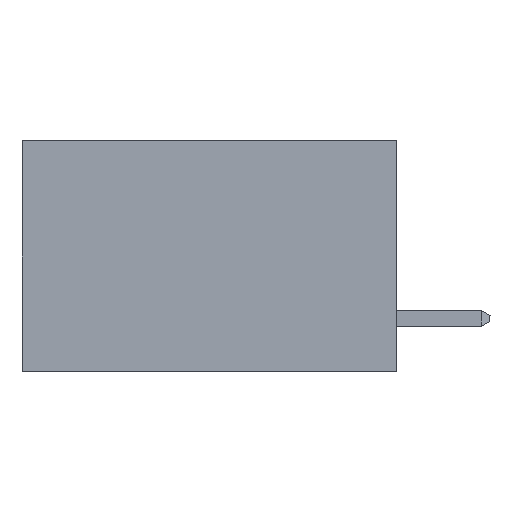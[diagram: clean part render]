
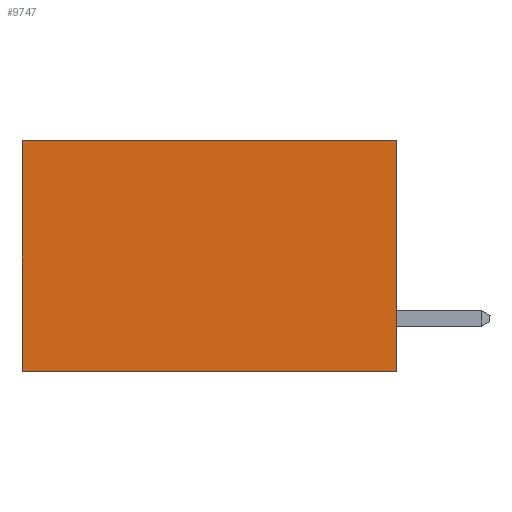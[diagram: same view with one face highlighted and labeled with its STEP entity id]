
A CAD part, left-side view. The second image highlights one B-rep face of the part: STEP entity #9747.
In plain terms, the highlighted planar face has unit normal (-1, 0, 0).
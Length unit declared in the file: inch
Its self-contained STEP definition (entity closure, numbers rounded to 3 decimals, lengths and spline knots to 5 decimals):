
#568 = PLANE ( 'NONE',  #11723 ) ;
#1338 = CARTESIAN_POINT ( 'NONE',  ( 0.2615, 0., -0.37 ) ) ;
#1835 = CARTESIAN_POINT ( 'NONE',  ( 0.2615, 0., -0.37 ) ) ;
#3425 = LINE ( 'NONE', #9785, #19022 ) ;
#3482 = EDGE_LOOP ( 'NONE', ( #17661, #17307, #8481, #19123 ) ) ;
#3510 = LINE ( 'NONE', #19877, #14342 ) ;
#6189 = LINE ( 'NONE', #20429, #20233 ) ;
#7108 = DIRECTION ( 'NONE',  ( 0., 0., -1. ) ) ;
#7297 = LINE ( 'NONE', #16811, #17138 ) ;
#7397 = DIRECTION ( 'NONE',  ( 0., 1., 0. ) ) ;
#8481 = ORIENTED_EDGE ( 'NONE', *, *, #20090, .F. ) ;
#8955 = CARTESIAN_POINT ( 'NONE',  ( 0.2615, 0.6, 0. ) ) ;
#9077 = VERTEX_POINT ( 'NONE', #9259 ) ;
#9109 = VERTEX_POINT ( 'NONE', #1338 ) ;
#9259 = CARTESIAN_POINT ( 'NONE',  ( 0.2615, 0.6, -0.37 ) ) ;
#9459 = DIRECTION ( 'NONE',  ( 0., 1., 0. ) ) ;
#9747 = ADVANCED_FACE ( 'NONE', ( #14953 ), #568, .F. ) ;
#9785 = CARTESIAN_POINT ( 'NONE',  ( 0.2615, 0.6, -0.37 ) ) ;
#10355 = DIRECTION ( 'NONE',  ( 0., 0., -1. ) ) ;
#10407 = EDGE_CURVE ( 'NONE', #12096, #12128, #7297, .T. ) ;
#11498 = DIRECTION ( 'NONE',  ( 0., 0., -1. ) ) ;
#11723 = AXIS2_PLACEMENT_3D ( 'NONE', #1835, #14551, #11498 ) ;
#12096 = VERTEX_POINT ( 'NONE', #13964 ) ;
#12128 = VERTEX_POINT ( 'NONE', #8955 ) ;
#13964 = CARTESIAN_POINT ( 'NONE',  ( 0.2615, 0., 0. ) ) ;
#14342 = VECTOR ( 'NONE', #7108, 39.37008 ) ;
#14551 = DIRECTION ( 'NONE',  ( 1., 0., 0. ) ) ;
#14953 = FACE_OUTER_BOUND ( 'NONE', #3482, .T. ) ;
#16381 = EDGE_CURVE ( 'NONE', #9109, #9077, #6189, .T. ) ;
#16811 = CARTESIAN_POINT ( 'NONE',  ( 0.2615, 0., 0. ) ) ;
#17138 = VECTOR ( 'NONE', #7397, 39.37008 ) ;
#17307 = ORIENTED_EDGE ( 'NONE', *, *, #16381, .F. ) ;
#17661 = ORIENTED_EDGE ( 'NONE', *, *, #19676, .T. ) ;
#19022 = VECTOR ( 'NONE', #10355, 39.37008 ) ;
#19123 = ORIENTED_EDGE ( 'NONE', *, *, #10407, .T. ) ;
#19676 = EDGE_CURVE ( 'NONE', #12128, #9077, #3425, .T. ) ;
#19877 = CARTESIAN_POINT ( 'NONE',  ( 0.2615, 0., -0.37 ) ) ;
#20090 = EDGE_CURVE ( 'NONE', #12096, #9109, #3510, .T. ) ;
#20233 = VECTOR ( 'NONE', #9459, 39.37008 ) ;
#20429 = CARTESIAN_POINT ( 'NONE',  ( 0.2615, 0., -0.37 ) ) ;
